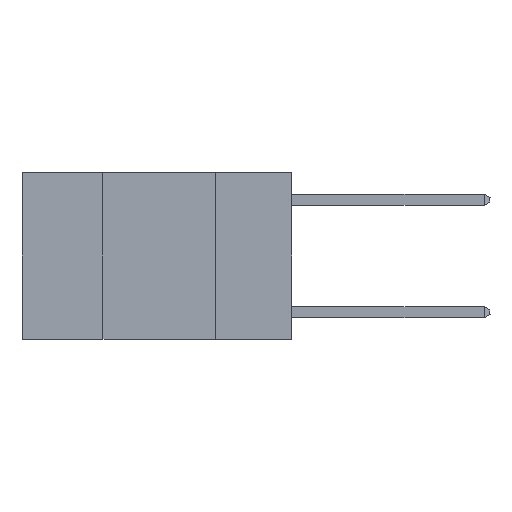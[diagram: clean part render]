
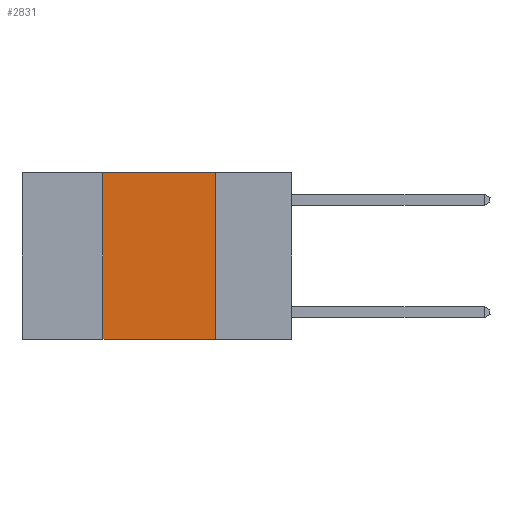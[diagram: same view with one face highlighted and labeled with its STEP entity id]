
A CAD part, left-side view. The second image highlights one B-rep face of the part: STEP entity #2831.
In plain terms, the highlighted planar face has unit normal (-1, 0, 0).
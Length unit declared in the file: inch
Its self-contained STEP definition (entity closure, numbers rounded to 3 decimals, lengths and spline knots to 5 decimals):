
#2831 = ADVANCED_FACE ( 'NONE', ( #5916 ), #11845, .F. ) ;
#2844 = CARTESIAN_POINT ( 'NONE',  ( 0., 0.6, -0.37 ) ) ;
#3122 = LINE ( 'NONE', #2844, #5456 ) ;
#3426 = CARTESIAN_POINT ( 'NONE',  ( 0., 0.42, 0. ) ) ;
#4388 = VERTEX_POINT ( 'NONE', #18561 ) ;
#5316 = CARTESIAN_POINT ( 'NONE',  ( 0., 0.42, 0. ) ) ;
#5456 = VECTOR ( 'NONE', #17173, 39.37008 ) ;
#5916 = FACE_OUTER_BOUND ( 'NONE', #13590, .T. ) ;
#6367 = ORIENTED_EDGE ( 'NONE', *, *, #14093, .T. ) ;
#7108 = LINE ( 'NONE', #3426, #19997 ) ;
#8453 = VERTEX_POINT ( 'NONE', #9415 ) ;
#9415 = CARTESIAN_POINT ( 'NONE',  ( 0., 0.42, -0.37 ) ) ;
#10171 = DIRECTION ( 'NONE',  ( 0., -1., 0. ) ) ;
#11071 = LINE ( 'NONE', #22982, #15775 ) ;
#11465 = CARTESIAN_POINT ( 'NONE',  ( 0., 0.17, -0.37 ) ) ;
#11845 = PLANE ( 'NONE',  #21745 ) ;
#11904 = VERTEX_POINT ( 'NONE', #11465 ) ;
#11974 = CARTESIAN_POINT ( 'NONE',  ( 0., 0.6, 0. ) ) ;
#12378 = DIRECTION ( 'NONE',  ( 0., 0., -1. ) ) ;
#13061 = DIRECTION ( 'NONE',  ( 0., 0., 1. ) ) ;
#13590 = EDGE_LOOP ( 'NONE', ( #22668, #17266, #22034, #6367 ) ) ;
#14093 = EDGE_CURVE ( 'NONE', #8453, #11904, #3122, .T. ) ;
#14234 = VERTEX_POINT ( 'NONE', #5316 ) ;
#15775 = VECTOR ( 'NONE', #21012, 39.37008 ) ;
#17173 = DIRECTION ( 'NONE',  ( 0., -1., 0. ) ) ;
#17266 = ORIENTED_EDGE ( 'NONE', *, *, #20246, .F. ) ;
#17783 = CARTESIAN_POINT ( 'NONE',  ( 0., 0.6, 0. ) ) ;
#18561 = CARTESIAN_POINT ( 'NONE',  ( 0., 0.17, 0. ) ) ;
#19984 = DIRECTION ( 'NONE',  ( 1., 0., 0. ) ) ;
#19997 = VECTOR ( 'NONE', #13061, 39.37008 ) ;
#20246 = EDGE_CURVE ( 'NONE', #14234, #4388, #23783, .T. ) ;
#21012 = DIRECTION ( 'NONE',  ( 0., 0., -1. ) ) ;
#21380 = VECTOR ( 'NONE', #10171, 39.37008 ) ;
#21745 = AXIS2_PLACEMENT_3D ( 'NONE', #11974, #19984, #12378 ) ;
#22034 = ORIENTED_EDGE ( 'NONE', *, *, #25747, .F. ) ;
#22198 = EDGE_CURVE ( 'NONE', #4388, #11904, #11071, .T. ) ;
#22668 = ORIENTED_EDGE ( 'NONE', *, *, #22198, .F. ) ;
#22982 = CARTESIAN_POINT ( 'NONE',  ( 0., 0.17, 0. ) ) ;
#23783 = LINE ( 'NONE', #17783, #21380 ) ;
#25747 = EDGE_CURVE ( 'NONE', #8453, #14234, #7108, .T. ) ;
